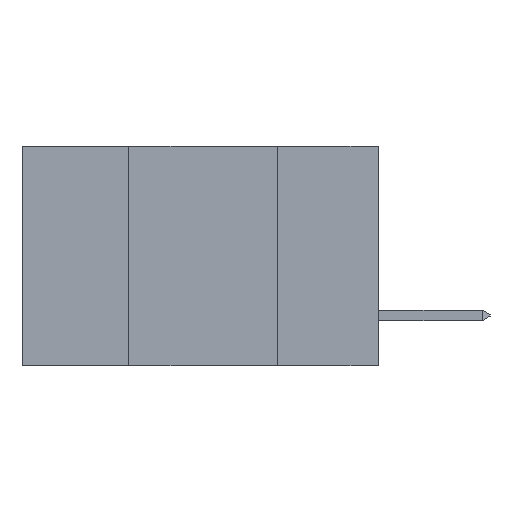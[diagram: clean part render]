
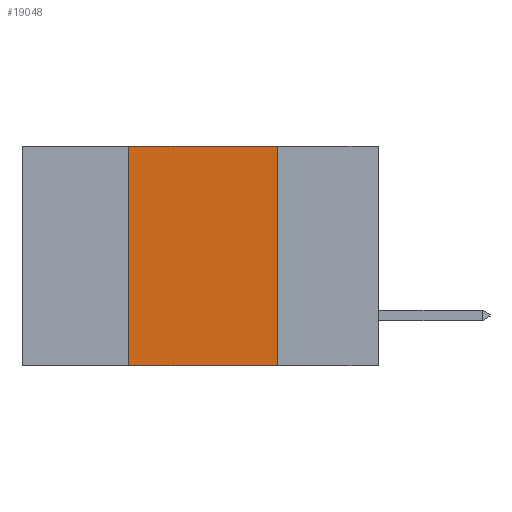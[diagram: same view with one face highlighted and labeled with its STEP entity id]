
A CAD part, left-side view. The second image highlights one B-rep face of the part: STEP entity #19048.
In plain terms, the highlighted planar face has unit normal (-1, 0, 0).
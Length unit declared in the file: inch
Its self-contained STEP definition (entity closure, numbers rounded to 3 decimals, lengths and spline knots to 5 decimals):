
#42 = EDGE_CURVE ( 'NONE', #10453, #15384, #19677, .T. ) ;
#1077 = EDGE_CURVE ( 'NONE', #15384, #14790, #14657, .T. ) ;
#1670 = DIRECTION ( 'NONE',  ( 0., 0., -1. ) ) ;
#1865 = CARTESIAN_POINT ( 'NONE',  ( 0., 0.6, -0.37 ) ) ;
#2131 = EDGE_CURVE ( 'NONE', #14790, #10149, #19153, .T. ) ;
#3877 = AXIS2_PLACEMENT_3D ( 'NONE', #17712, #8645, #19100 ) ;
#3915 = PLANE ( 'NONE',  #3877 ) ;
#5043 = EDGE_LOOP ( 'NONE', ( #6083, #17522, #17075, #16620 ) ) ;
#5222 = CARTESIAN_POINT ( 'NONE',  ( 0., 0.42, -0.37 ) ) ;
#5983 = CARTESIAN_POINT ( 'NONE',  ( 0., 0.17, -0.37 ) ) ;
#6083 = ORIENTED_EDGE ( 'NONE', *, *, #2131, .F. ) ;
#6488 = VECTOR ( 'NONE', #15991, 39.37008 ) ;
#7838 = VECTOR ( 'NONE', #9606, 39.37008 ) ;
#8001 = CARTESIAN_POINT ( 'NONE',  ( 0., 0.42, 0. ) ) ;
#8326 = LINE ( 'NONE', #1865, #7838 ) ;
#8645 = DIRECTION ( 'NONE',  ( 1., 0., 0. ) ) ;
#9606 = DIRECTION ( 'NONE',  ( 0., -1., 0. ) ) ;
#10081 = DIRECTION ( 'NONE',  ( 0., 0., 1. ) ) ;
#10149 = VERTEX_POINT ( 'NONE', #11569 ) ;
#10453 = VERTEX_POINT ( 'NONE', #19595 ) ;
#11569 = CARTESIAN_POINT ( 'NONE',  ( 0., 0.17, -0.37 ) ) ;
#14657 = LINE ( 'NONE', #18781, #6488 ) ;
#14790 = VERTEX_POINT ( 'NONE', #17261 ) ;
#15384 = VERTEX_POINT ( 'NONE', #8001 ) ;
#15892 = VECTOR ( 'NONE', #10081, 39.37008 ) ;
#15991 = DIRECTION ( 'NONE',  ( 0., -1., 0. ) ) ;
#16620 = ORIENTED_EDGE ( 'NONE', *, *, #18815, .T. ) ;
#17075 = ORIENTED_EDGE ( 'NONE', *, *, #42, .F. ) ;
#17261 = CARTESIAN_POINT ( 'NONE',  ( 0., 0.17, 0. ) ) ;
#17522 = ORIENTED_EDGE ( 'NONE', *, *, #1077, .F. ) ;
#17712 = CARTESIAN_POINT ( 'NONE',  ( 0., 0.6, 0. ) ) ;
#18727 = VECTOR ( 'NONE', #1670, 39.37008 ) ;
#18781 = CARTESIAN_POINT ( 'NONE',  ( 0., 0.6, 0. ) ) ;
#18815 = EDGE_CURVE ( 'NONE', #10453, #10149, #8326, .T. ) ;
#19048 = ADVANCED_FACE ( 'NONE', ( #19535 ), #3915, .F. ) ;
#19100 = DIRECTION ( 'NONE',  ( 0., 0., -1. ) ) ;
#19153 = LINE ( 'NONE', #5983, #18727 ) ;
#19535 = FACE_OUTER_BOUND ( 'NONE', #5043, .T. ) ;
#19595 = CARTESIAN_POINT ( 'NONE',  ( 0., 0.42, -0.37 ) ) ;
#19677 = LINE ( 'NONE', #5222, #15892 ) ;
